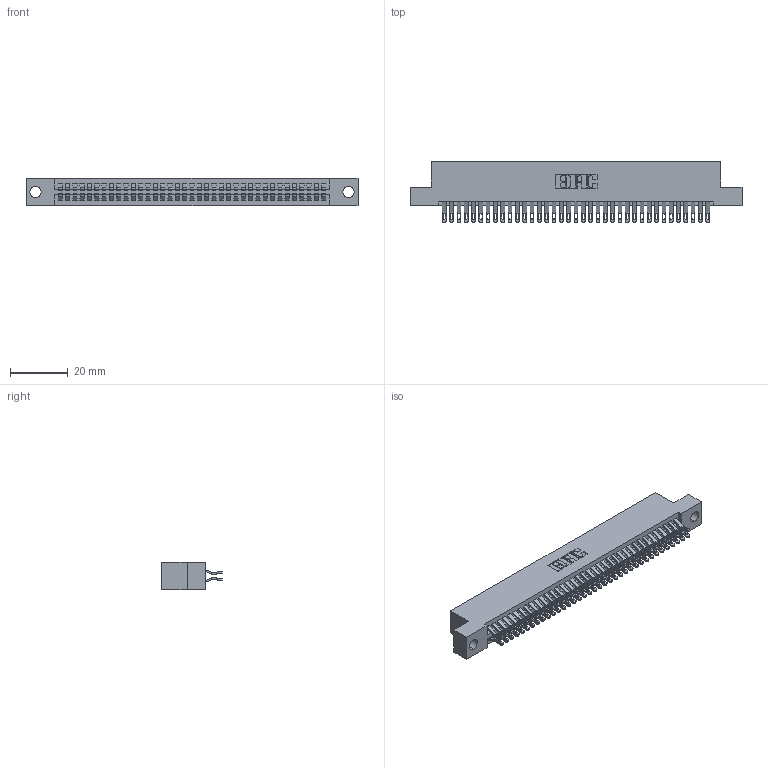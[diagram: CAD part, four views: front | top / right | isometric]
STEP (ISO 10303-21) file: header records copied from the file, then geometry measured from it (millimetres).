
FILE_DESCRIPTION (( 'STEP AP203' ), '1' );
FILE_NAME ('395-074-555-204.STEP', '2021-06-17T05:37:49', ( '' ), ( '' ), 'SwSTEP 2.0', 'SolidWorks 2020', '' );
FILE_SCHEMA (( 'CONFIG_CONTROL_DESIGN' ));
Length unit declared in the file: inch
Products named in the file (3): 395-074-555-204; 345-292-001_555 Tail; 345 Part_Flush Mounting Lugs - 0.156 Dia-TI
Assembly tree (75 placements, depth 2):
  395-074-555-204
    345 Part_Flush Mounting Lugs - 0.156 Dia-TI
    345-292-001_555 Tail  x74
Bounding box: 115.19 x 21.13 x 9.4 mm (x, y, z)
Volume: 11251.9 mm3; surface area: 17133.4 mm2
Topology: 75 solids, 75 shells, 4284 faces, 13475 edges, 8982 vertices
Faces by surface type: plane 2388, cylinder 1896
Entity records: 30449 total; most frequent: CARTESIAN_POINT 5148, ORIENTED_EDGE 5050, DIRECTION 4513, EDGE_CURVE 2525, LINE 2225, VECTOR 2225, VERTEX_POINT 1682, AXIS2_PLACEMENT_3D 1144
